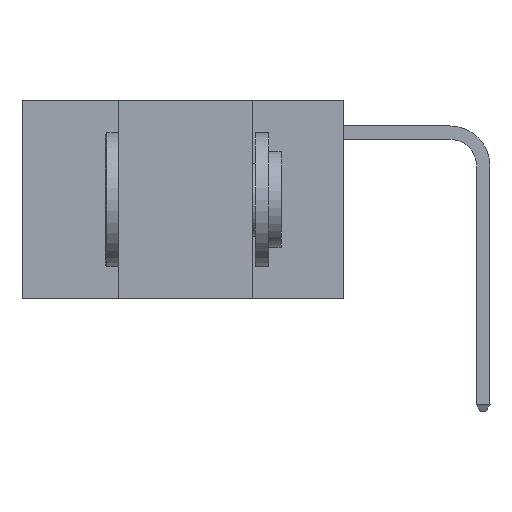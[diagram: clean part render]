
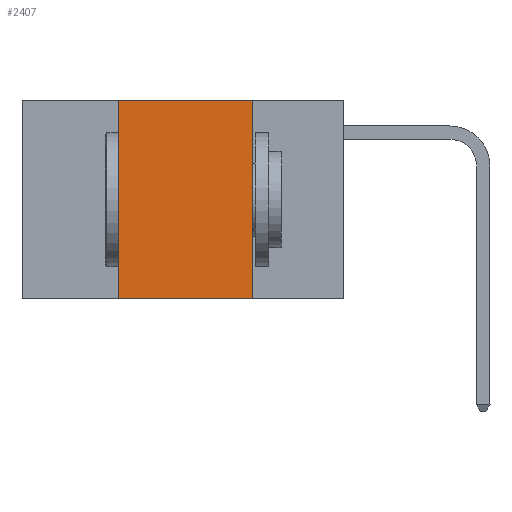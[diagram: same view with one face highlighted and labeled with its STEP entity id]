
A CAD part, left-side view. The second image highlights one B-rep face of the part: STEP entity #2407.
In plain terms, the highlighted planar face has unit normal (-1, 0, 0).
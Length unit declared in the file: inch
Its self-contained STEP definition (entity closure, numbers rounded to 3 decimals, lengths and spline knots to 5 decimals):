
#1243 = CARTESIAN_POINT ( 'NONE',  ( 0., 0.17, 0. ) ) ;
#2407 = ADVANCED_FACE ( 'NONE', ( #9877 ), #17297, .F. ) ;
#2761 = CARTESIAN_POINT ( 'NONE',  ( 0., 0.6, 0. ) ) ;
#2849 = LINE ( 'NONE', #18501, #14847 ) ;
#2966 = EDGE_CURVE ( 'NONE', #9282, #8360, #4160, .T. ) ;
#2996 = EDGE_CURVE ( 'NONE', #6087, #15340, #2849, .T. ) ;
#4131 = LINE ( 'NONE', #1243, #13822 ) ;
#4160 = LINE ( 'NONE', #2761, #10785 ) ;
#4185 = DIRECTION ( 'NONE',  ( 0., 0., -1. ) ) ;
#4235 = DIRECTION ( 'NONE',  ( 0., 0., -1. ) ) ;
#4290 = CARTESIAN_POINT ( 'NONE',  ( 0., 0.6, 0. ) ) ;
#5317 = CARTESIAN_POINT ( 'NONE',  ( 0., 0.42, 0. ) ) ;
#5804 = DIRECTION ( 'NONE',  ( 1., 0., 0. ) ) ;
#6087 = VERTEX_POINT ( 'NONE', #9351 ) ;
#6456 = AXIS2_PLACEMENT_3D ( 'NONE', #4290, #5804, #4185 ) ;
#8360 = VERTEX_POINT ( 'NONE', #16663 ) ;
#8667 = CARTESIAN_POINT ( 'NONE',  ( 0., 0.42, 0. ) ) ;
#9282 = VERTEX_POINT ( 'NONE', #8667 ) ;
#9351 = CARTESIAN_POINT ( 'NONE',  ( 0., 0.42, -0.37 ) ) ;
#9578 = LINE ( 'NONE', #5317, #14083 ) ;
#9850 = DIRECTION ( 'NONE',  ( 0., -1., 0. ) ) ;
#9877 = FACE_OUTER_BOUND ( 'NONE', #12791, .T. ) ;
#9916 = ORIENTED_EDGE ( 'NONE', *, *, #2966, .F. ) ;
#10785 = VECTOR ( 'NONE', #9850, 39.37008 ) ;
#11410 = EDGE_CURVE ( 'NONE', #6087, #9282, #9578, .T. ) ;
#11951 = ORIENTED_EDGE ( 'NONE', *, *, #2996, .T. ) ;
#12177 = EDGE_CURVE ( 'NONE', #8360, #15340, #4131, .T. ) ;
#12791 = EDGE_LOOP ( 'NONE', ( #14191, #9916, #13211, #11951 ) ) ;
#13211 = ORIENTED_EDGE ( 'NONE', *, *, #11410, .F. ) ;
#13717 = DIRECTION ( 'NONE',  ( 0., 0., 1. ) ) ;
#13822 = VECTOR ( 'NONE', #4235, 39.37008 ) ;
#14083 = VECTOR ( 'NONE', #13717, 39.37008 ) ;
#14191 = ORIENTED_EDGE ( 'NONE', *, *, #12177, .F. ) ;
#14847 = VECTOR ( 'NONE', #18314, 39.37008 ) ;
#14959 = CARTESIAN_POINT ( 'NONE',  ( 0., 0.17, -0.37 ) ) ;
#15340 = VERTEX_POINT ( 'NONE', #14959 ) ;
#16663 = CARTESIAN_POINT ( 'NONE',  ( 0., 0.17, 0. ) ) ;
#17297 = PLANE ( 'NONE',  #6456 ) ;
#18314 = DIRECTION ( 'NONE',  ( 0., -1., 0. ) ) ;
#18501 = CARTESIAN_POINT ( 'NONE',  ( 0., 0.6, -0.37 ) ) ;
